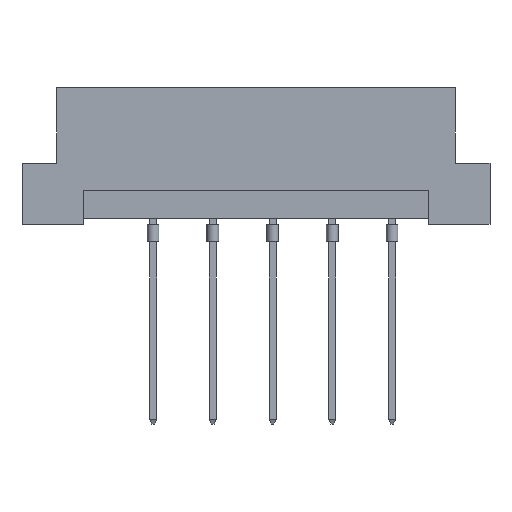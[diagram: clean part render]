
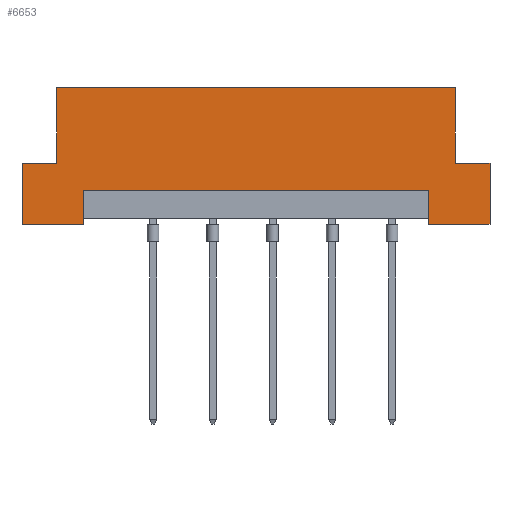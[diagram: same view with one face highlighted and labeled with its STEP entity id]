
A CAD part, front view. The second image highlights one B-rep face of the part: STEP entity #6653.
In plain terms, the highlighted planar face has unit normal (0, -1, 0).
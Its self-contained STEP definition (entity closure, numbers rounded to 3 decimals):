
#22 = VERTEX_POINT ( 'NONE', #1718 ) ;
#74 = ORIENTED_EDGE ( 'NONE', *, *, #1072, .F. ) ;
#184 = LINE ( 'NONE', #4973, #2853 ) ;
#238 = ORIENTED_EDGE ( 'NONE', *, *, #4301, .F. ) ;
#344 = VECTOR ( 'NONE', #5623, 1000. ) ;
#535 = CARTESIAN_POINT ( 'NONE',  ( 14.69, 0., 0.5 ) ) ;
#618 = DIRECTION ( 'NONE',  ( 0., 0., 1. ) ) ;
#710 = ORIENTED_EDGE ( 'NONE', *, *, #1039, .F. ) ;
#764 = CARTESIAN_POINT ( 'NONE',  ( 19.9, 0., 5.2 ) ) ;
#958 = CARTESIAN_POINT ( 'NONE',  ( 14.69, 0., 2.9 ) ) ;
#998 = DIRECTION ( 'NONE',  ( -1., 0., 0. ) ) ;
#1039 = EDGE_CURVE ( 'NONE', #3831, #5633, #5309, .T. ) ;
#1072 = EDGE_CURVE ( 'NONE', #1665, #3979, #7034, .T. ) ;
#1074 = EDGE_CURVE ( 'NONE', #1229, #6474, #2650, .T. ) ;
#1220 = CARTESIAN_POINT ( 'NONE',  ( 19.9, 0., 5.2 ) ) ;
#1229 = VERTEX_POINT ( 'NONE', #3447 ) ;
#1257 = CARTESIAN_POINT ( 'NONE',  ( 16.94, 0., 11.6 ) ) ;
#1361 = VECTOR ( 'NONE', #998, 1000. ) ;
#1423 = CARTESIAN_POINT ( 'NONE',  ( -14.69, 0., 2.9 ) ) ;
#1458 = LINE ( 'NONE', #6478, #2396 ) ;
#1474 = CARTESIAN_POINT ( 'NONE',  ( -19.9, 0., 0. ) ) ;
#1538 = DIRECTION ( 'NONE',  ( -1., 0., 0. ) ) ;
#1581 = CARTESIAN_POINT ( 'NONE',  ( -14.69, 0., 0.5 ) ) ;
#1636 = DIRECTION ( 'NONE',  ( 0., 0., -1. ) ) ;
#1639 = VERTEX_POINT ( 'NONE', #7027 ) ;
#1664 = EDGE_CURVE ( 'NONE', #3831, #22, #2245, .T. ) ;
#1665 = VERTEX_POINT ( 'NONE', #1220 ) ;
#1686 = ORIENTED_EDGE ( 'NONE', *, *, #5326, .F. ) ;
#1718 = CARTESIAN_POINT ( 'NONE',  ( 14.69, 0., 0. ) ) ;
#1744 = CARTESIAN_POINT ( 'NONE',  ( 14.69, 0., 2.9 ) ) ;
#1755 = LINE ( 'NONE', #5556, #5936 ) ;
#1827 = AXIS2_PLACEMENT_3D ( 'NONE', #5771, #4653, #6849 ) ;
#2116 = VERTEX_POINT ( 'NONE', #3348 ) ;
#2245 = LINE ( 'NONE', #535, #4721 ) ;
#2396 = VECTOR ( 'NONE', #3649, 1000. ) ;
#2650 = LINE ( 'NONE', #2679, #6077 ) ;
#2656 = ORIENTED_EDGE ( 'NONE', *, *, #2997, .F. ) ;
#2679 = CARTESIAN_POINT ( 'NONE',  ( -19.9, 0., 11.6 ) ) ;
#2853 = VECTOR ( 'NONE', #6009, 1000. ) ;
#2997 = EDGE_CURVE ( 'NONE', #3979, #22, #3436, .T. ) ;
#3090 = LINE ( 'NONE', #1474, #5024 ) ;
#3093 = VECTOR ( 'NONE', #1538, 1000. ) ;
#3224 = ORIENTED_EDGE ( 'NONE', *, *, #1664, .T. ) ;
#3324 = LINE ( 'NONE', #764, #6617 ) ;
#3348 = CARTESIAN_POINT ( 'NONE',  ( 16.94, 0., 5.2 ) ) ;
#3436 = LINE ( 'NONE', #6086, #344 ) ;
#3447 = CARTESIAN_POINT ( 'NONE',  ( -16.94, 0., 11.6 ) ) ;
#3542 = CARTESIAN_POINT ( 'NONE',  ( -14.69, 0., 0. ) ) ;
#3649 = DIRECTION ( 'NONE',  ( 1., 0., 0. ) ) ;
#3717 = CARTESIAN_POINT ( 'NONE',  ( -19.9, 0., 0. ) ) ;
#3831 = VERTEX_POINT ( 'NONE', #1744 ) ;
#3945 = VERTEX_POINT ( 'NONE', #3542 ) ;
#3979 = VERTEX_POINT ( 'NONE', #5624 ) ;
#4084 = VERTEX_POINT ( 'NONE', #5324 ) ;
#4087 = EDGE_CURVE ( 'NONE', #3945, #4084, #7047, .T. ) ;
#4239 = DIRECTION ( 'NONE',  ( 1., 0., 0. ) ) ;
#4301 = EDGE_CURVE ( 'NONE', #4084, #5608, #3090, .T. ) ;
#4306 = LINE ( 'NONE', #1581, #5263 ) ;
#4336 = ORIENTED_EDGE ( 'NONE', *, *, #4610, .F. ) ;
#4610 = EDGE_CURVE ( 'NONE', #1639, #1229, #1755, .T. ) ;
#4653 = DIRECTION ( 'NONE',  ( 0., 1., 0. ) ) ;
#4721 = VECTOR ( 'NONE', #1636, 1000. ) ;
#4774 = ORIENTED_EDGE ( 'NONE', *, *, #1074, .F. ) ;
#4849 = ORIENTED_EDGE ( 'NONE', *, *, #5114, .T. ) ;
#4973 = CARTESIAN_POINT ( 'NONE',  ( 16.94, 0., 5.2 ) ) ;
#5024 = VECTOR ( 'NONE', #5276, 1000. ) ;
#5114 = EDGE_CURVE ( 'NONE', #2116, #6474, #184, .T. ) ;
#5193 = PLANE ( 'NONE',  #1827 ) ;
#5249 = DIRECTION ( 'NONE',  ( 0., 0., -1. ) ) ;
#5263 = VECTOR ( 'NONE', #5249, 1000. ) ;
#5276 = DIRECTION ( 'NONE',  ( 0., 0., 1. ) ) ;
#5309 = LINE ( 'NONE', #958, #3093 ) ;
#5324 = CARTESIAN_POINT ( 'NONE',  ( -19.9, 0., 0. ) ) ;
#5326 = EDGE_CURVE ( 'NONE', #5608, #1639, #1458, .T. ) ;
#5413 = CARTESIAN_POINT ( 'NONE',  ( 19.9, 0., 0. ) ) ;
#5556 = CARTESIAN_POINT ( 'NONE',  ( -16.94, 0., 5.2 ) ) ;
#5566 = ORIENTED_EDGE ( 'NONE', *, *, #6459, .F. ) ;
#5608 = VERTEX_POINT ( 'NONE', #6614 ) ;
#5623 = DIRECTION ( 'NONE',  ( -1., 0., 0. ) ) ;
#5624 = CARTESIAN_POINT ( 'NONE',  ( 19.9, 0., 0. ) ) ;
#5633 = VERTEX_POINT ( 'NONE', #1423 ) ;
#5760 = ORIENTED_EDGE ( 'NONE', *, *, #5963, .F. ) ;
#5771 = CARTESIAN_POINT ( 'NONE',  ( -19.9, 0., 11.6 ) ) ;
#5936 = VECTOR ( 'NONE', #618, 1000. ) ;
#5963 = EDGE_CURVE ( 'NONE', #5633, #3945, #4306, .T. ) ;
#6009 = DIRECTION ( 'NONE',  ( 0., 0., 1. ) ) ;
#6077 = VECTOR ( 'NONE', #4239, 1000. ) ;
#6086 = CARTESIAN_POINT ( 'NONE',  ( -19.9, 0., 0. ) ) ;
#6153 = ORIENTED_EDGE ( 'NONE', *, *, #4087, .F. ) ;
#6434 = DIRECTION ( 'NONE',  ( 0., 0., -1. ) ) ;
#6459 = EDGE_CURVE ( 'NONE', #2116, #1665, #3324, .T. ) ;
#6474 = VERTEX_POINT ( 'NONE', #1257 ) ;
#6478 = CARTESIAN_POINT ( 'NONE',  ( -19.9, 0., 5.2 ) ) ;
#6604 = EDGE_LOOP ( 'NONE', ( #710, #3224, #2656, #74, #5566, #4849, #4774, #4336, #1686, #238, #6153, #5760 ) ) ;
#6614 = CARTESIAN_POINT ( 'NONE',  ( -19.9, 0., 5.2 ) ) ;
#6617 = VECTOR ( 'NONE', #6664, 1000. ) ;
#6653 = ADVANCED_FACE ( 'NONE', ( #6816 ), #5193, .F. ) ;
#6664 = DIRECTION ( 'NONE',  ( 1., 0., 0. ) ) ;
#6773 = VECTOR ( 'NONE', #6434, 1000. ) ;
#6816 = FACE_OUTER_BOUND ( 'NONE', #6604, .T. ) ;
#6849 = DIRECTION ( 'NONE',  ( 0., 0., 1. ) ) ;
#7027 = CARTESIAN_POINT ( 'NONE',  ( -16.94, 0., 5.2 ) ) ;
#7034 = LINE ( 'NONE', #5413, #6773 ) ;
#7047 = LINE ( 'NONE', #3717, #1361 ) ;
